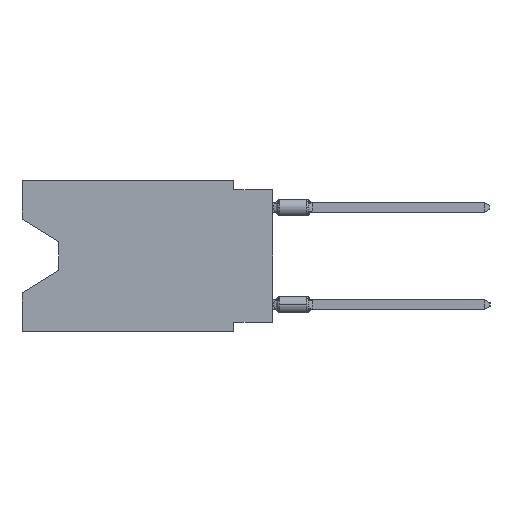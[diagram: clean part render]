
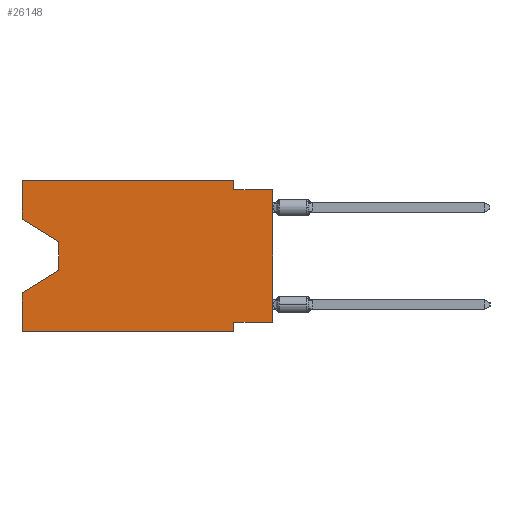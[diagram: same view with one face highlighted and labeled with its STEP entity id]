
A CAD part, left-side view. The second image highlights one B-rep face of the part: STEP entity #26148.
In plain terms, the highlighted planar face has unit normal (-1, 0, 0).
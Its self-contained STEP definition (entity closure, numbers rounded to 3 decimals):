
#933 = ORIENTED_EDGE ( 'NONE', *, *, #60565, .F. ) ;
#1926 = VECTOR ( 'NONE', #3678, 1000. ) ;
#2586 = LINE ( 'NONE', #59706, #52542 ) ;
#2665 = VECTOR ( 'NONE', #57590, 1000. ) ;
#3678 = DIRECTION ( 'NONE',  ( 0., -0.855, -0.519 ) ) ;
#5036 = ORIENTED_EDGE ( 'NONE', *, *, #47333, .F. ) ;
#5484 = CARTESIAN_POINT ( 'NONE',  ( 0., 0., -0.635 ) ) ;
#5699 = VERTEX_POINT ( 'NONE', #10034 ) ;
#6106 = ORIENTED_EDGE ( 'NONE', *, *, #12132, .T. ) ;
#6211 = DIRECTION ( 'NONE',  ( 0., 0., -1. ) ) ;
#6609 = VECTOR ( 'NONE', #7372, 1000. ) ;
#6775 = VERTEX_POINT ( 'NONE', #54964 ) ;
#6882 = VERTEX_POINT ( 'NONE', #13803 ) ;
#7168 = DIRECTION ( 'NONE',  ( 0., 0.855, -0.519 ) ) ;
#7372 = DIRECTION ( 'NONE',  ( 0., 0., -1. ) ) ;
#7547 = DIRECTION ( 'NONE',  ( 0., 0., -1. ) ) ;
#8109 = LINE ( 'NONE', #32925, #22936 ) ;
#9578 = VECTOR ( 'NONE', #12169, 1000. ) ;
#9965 = ORIENTED_EDGE ( 'NONE', *, *, #38330, .T. ) ;
#10034 = CARTESIAN_POINT ( 'NONE',  ( 0., 13.97, -5.893 ) ) ;
#11317 = EDGE_CURVE ( 'NONE', #26369, #6775, #31649, .T. ) ;
#11362 = DIRECTION ( 'NONE',  ( 0., 1., 0. ) ) ;
#12132 = EDGE_CURVE ( 'NONE', #19300, #5699, #61028, .T. ) ;
#12169 = DIRECTION ( 'NONE',  ( 0., 0., 1. ) ) ;
#12824 = EDGE_CURVE ( 'NONE', #23094, #31410, #59338, .T. ) ;
#12985 = DIRECTION ( 'NONE',  ( 0., -1., 0. ) ) ;
#13090 = CARTESIAN_POINT ( 'NONE',  ( 0., 16.383, 0. ) ) ;
#13803 = CARTESIAN_POINT ( 'NONE',  ( 0., 2.54, -9.271 ) ) ;
#13960 = LINE ( 'NONE', #5484, #2665 ) ;
#14608 = EDGE_CURVE ( 'NONE', #5699, #6775, #55808, .T. ) ;
#14709 = VECTOR ( 'NONE', #7168, 1000. ) ;
#15385 = CARTESIAN_POINT ( 'NONE',  ( 0., 16.383, 0. ) ) ;
#15690 = VECTOR ( 'NONE', #34880, 1000. ) ;
#15721 = DIRECTION ( 'NONE',  ( 0., 0., -1. ) ) ;
#16034 = CARTESIAN_POINT ( 'NONE',  ( 0., 2.54, -9.906 ) ) ;
#17513 = AXIS2_PLACEMENT_3D ( 'NONE', #27943, #18179, #7547 ) ;
#17813 = VECTOR ( 'NONE', #15721, 1000. ) ;
#18179 = DIRECTION ( 'NONE',  ( 1., 0., 0. ) ) ;
#19209 = LINE ( 'NONE', #22985, #36071 ) ;
#19300 = VERTEX_POINT ( 'NONE', #45665 ) ;
#21008 = VECTOR ( 'NONE', #33929, 1000. ) ;
#21349 = LINE ( 'NONE', #54337, #17813 ) ;
#21548 = LINE ( 'NONE', #49497, #54489 ) ;
#21820 = CARTESIAN_POINT ( 'NONE',  ( 0., 16.383, -9.906 ) ) ;
#22420 = ORIENTED_EDGE ( 'NONE', *, *, #59574, .T. ) ;
#22936 = VECTOR ( 'NONE', #26960, 1000. ) ;
#22985 = CARTESIAN_POINT ( 'NONE',  ( 0., 16.383, -9.906 ) ) ;
#23094 = VERTEX_POINT ( 'NONE', #58651 ) ;
#26148 = ADVANCED_FACE ( 'NONE', ( #41152 ), #27635, .F. ) ;
#26369 = VERTEX_POINT ( 'NONE', #21820 ) ;
#26960 = DIRECTION ( 'NONE',  ( 0., 0., 1. ) ) ;
#27256 = CARTESIAN_POINT ( 'NONE',  ( 0., 13.97, -5.893 ) ) ;
#27511 = ORIENTED_EDGE ( 'NONE', *, *, #60045, .T. ) ;
#27635 = PLANE ( 'NONE',  #17513 ) ;
#27943 = CARTESIAN_POINT ( 'NONE',  ( 0., 16.383, 0. ) ) ;
#30704 = CARTESIAN_POINT ( 'NONE',  ( 0., 2.54, 0. ) ) ;
#31410 = VERTEX_POINT ( 'NONE', #13090 ) ;
#31638 = ORIENTED_EDGE ( 'NONE', *, *, #44890, .F. ) ;
#31649 = LINE ( 'NONE', #58944, #9578 ) ;
#31767 = ORIENTED_EDGE ( 'NONE', *, *, #12824, .F. ) ;
#32795 = VERTEX_POINT ( 'NONE', #61118 ) ;
#32925 = CARTESIAN_POINT ( 'NONE',  ( 0., 0., 0. ) ) ;
#33929 = DIRECTION ( 'NONE',  ( 0., -1., 0. ) ) ;
#34236 = LINE ( 'NONE', #53352, #21008 ) ;
#34880 = DIRECTION ( 'NONE',  ( 0., 0., 1. ) ) ;
#34936 = EDGE_CURVE ( 'NONE', #42059, #32795, #21349, .T. ) ;
#35721 = CARTESIAN_POINT ( 'NONE',  ( 0., 16.383, -2.546 ) ) ;
#36071 = VECTOR ( 'NONE', #12985, 1000. ) ;
#37208 = ORIENTED_EDGE ( 'NONE', *, *, #11317, .F. ) ;
#38330 = EDGE_CURVE ( 'NONE', #23094, #19300, #45752, .T. ) ;
#40064 = ORIENTED_EDGE ( 'NONE', *, *, #42072, .F. ) ;
#40661 = VERTEX_POINT ( 'NONE', #61702 ) ;
#41152 = FACE_OUTER_BOUND ( 'NONE', #59334, .T. ) ;
#42059 = VERTEX_POINT ( 'NONE', #30704 ) ;
#42072 = EDGE_CURVE ( 'NONE', #6882, #59089, #21548, .T. ) ;
#44890 = EDGE_CURVE ( 'NONE', #40661, #6882, #2586, .T. ) ;
#45665 = CARTESIAN_POINT ( 'NONE',  ( 0., 13.97, -4.013 ) ) ;
#45752 = LINE ( 'NONE', #35721, #1926 ) ;
#45991 = CARTESIAN_POINT ( 'NONE',  ( 0., 13.97, -4.013 ) ) ;
#47333 = EDGE_CURVE ( 'NONE', #32795, #59783, #13960, .T. ) ;
#49497 = CARTESIAN_POINT ( 'NONE',  ( 0., 2.54, -9.906 ) ) ;
#52542 = VECTOR ( 'NONE', #11362, 1000. ) ;
#53352 = CARTESIAN_POINT ( 'NONE',  ( 0., 16.383, 0. ) ) ;
#54121 = CARTESIAN_POINT ( 'NONE',  ( 0., 0., -0.635 ) ) ;
#54337 = CARTESIAN_POINT ( 'NONE',  ( 0., 2.54, 0. ) ) ;
#54372 = ORIENTED_EDGE ( 'NONE', *, *, #34936, .F. ) ;
#54489 = VECTOR ( 'NONE', #6211, 1000. ) ;
#54964 = CARTESIAN_POINT ( 'NONE',  ( 0., 16.383, -7.36 ) ) ;
#55808 = LINE ( 'NONE', #27256, #14709 ) ;
#57590 = DIRECTION ( 'NONE',  ( 0., -1., 0. ) ) ;
#58517 = ORIENTED_EDGE ( 'NONE', *, *, #14608, .T. ) ;
#58651 = CARTESIAN_POINT ( 'NONE',  ( 0., 16.383, -2.546 ) ) ;
#58944 = CARTESIAN_POINT ( 'NONE',  ( 0., 16.383, 0. ) ) ;
#59089 = VERTEX_POINT ( 'NONE', #16034 ) ;
#59334 = EDGE_LOOP ( 'NONE', ( #9965, #6106, #58517, #37208, #27511, #40064, #31638, #22420, #5036, #54372, #933, #31767 ) ) ;
#59338 = LINE ( 'NONE', #15385, #15690 ) ;
#59574 = EDGE_CURVE ( 'NONE', #40661, #59783, #8109, .T. ) ;
#59706 = CARTESIAN_POINT ( 'NONE',  ( 0., 0., -9.271 ) ) ;
#59783 = VERTEX_POINT ( 'NONE', #54121 ) ;
#60045 = EDGE_CURVE ( 'NONE', #26369, #59089, #19209, .T. ) ;
#60565 = EDGE_CURVE ( 'NONE', #31410, #42059, #34236, .T. ) ;
#61028 = LINE ( 'NONE', #45991, #6609 ) ;
#61118 = CARTESIAN_POINT ( 'NONE',  ( 0., 2.54, -0.635 ) ) ;
#61702 = CARTESIAN_POINT ( 'NONE',  ( 0., 0., -9.271 ) ) ;
